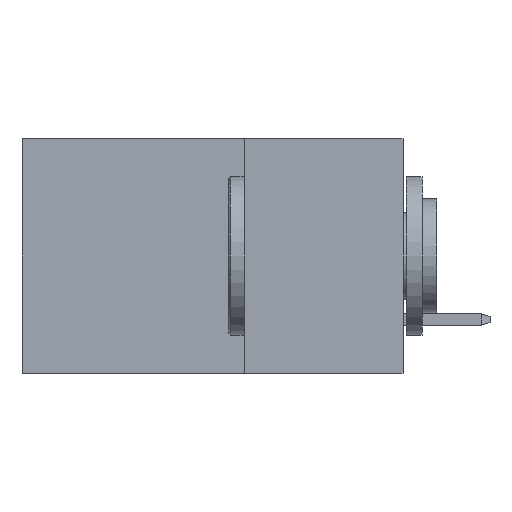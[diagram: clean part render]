
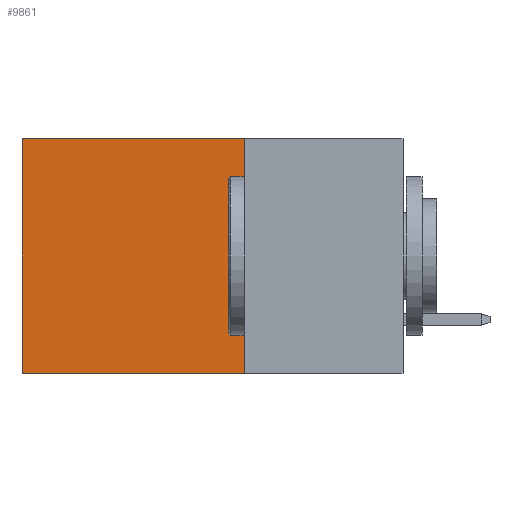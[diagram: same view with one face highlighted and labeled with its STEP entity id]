
A CAD part, left-side view. The second image highlights one B-rep face of the part: STEP entity #9861.
In plain terms, the highlighted planar face has unit normal (-1, 0, 0).
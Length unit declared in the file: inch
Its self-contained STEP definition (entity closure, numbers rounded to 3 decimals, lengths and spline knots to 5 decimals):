
#599 = VERTEX_POINT ( 'NONE', #4474 ) ;
#814 = CARTESIAN_POINT ( 'NONE',  ( 0.2875, 0.25, 0. ) ) ;
#1584 = CARTESIAN_POINT ( 'NONE',  ( 0.2875, 0.6, -0.37 ) ) ;
#2163 = DIRECTION ( 'NONE',  ( 0., 0., -1. ) ) ;
#2333 = LINE ( 'NONE', #814, #4187 ) ;
#2511 = DIRECTION ( 'NONE',  ( 0., 0., -1. ) ) ;
#2760 = CARTESIAN_POINT ( 'NONE',  ( 0.2875, 0.25, 0. ) ) ;
#2828 = EDGE_LOOP ( 'NONE', ( #7615, #7182, #3556, #6015 ) ) ;
#2941 = DIRECTION ( 'NONE',  ( 1., 0., 0. ) ) ;
#2967 = DIRECTION ( 'NONE',  ( 0., 1., 0. ) ) ;
#3556 = ORIENTED_EDGE ( 'NONE', *, *, #6096, .F. ) ;
#3710 = AXIS2_PLACEMENT_3D ( 'NONE', #10039, #2941, #2163 ) ;
#4136 = CARTESIAN_POINT ( 'NONE',  ( 0.2875, 0.6, 0. ) ) ;
#4187 = VECTOR ( 'NONE', #6932, 39.37008 ) ;
#4474 = CARTESIAN_POINT ( 'NONE',  ( 0.2875, 0.25, -0.37 ) ) ;
#4625 = VERTEX_POINT ( 'NONE', #6650 ) ;
#5162 = CARTESIAN_POINT ( 'NONE',  ( 0.2875, 0.6, 0. ) ) ;
#5188 = FACE_OUTER_BOUND ( 'NONE', #2828, .T. ) ;
#5555 = VERTEX_POINT ( 'NONE', #5162 ) ;
#5666 = VECTOR ( 'NONE', #9142, 39.37008 ) ;
#5919 = EDGE_CURVE ( 'NONE', #4625, #5555, #8323, .T. ) ;
#6015 = ORIENTED_EDGE ( 'NONE', *, *, #5919, .T. ) ;
#6096 = EDGE_CURVE ( 'NONE', #4625, #599, #2333, .T. ) ;
#6650 = CARTESIAN_POINT ( 'NONE',  ( 0.2875, 0.25, 0. ) ) ;
#6917 = LINE ( 'NONE', #4136, #7643 ) ;
#6932 = DIRECTION ( 'NONE',  ( 0., 0., -1. ) ) ;
#6945 = CARTESIAN_POINT ( 'NONE',  ( 0.2875, 0.25, -0.37 ) ) ;
#7068 = VERTEX_POINT ( 'NONE', #1584 ) ;
#7182 = ORIENTED_EDGE ( 'NONE', *, *, #8668, .F. ) ;
#7501 = PLANE ( 'NONE',  #3710 ) ;
#7615 = ORIENTED_EDGE ( 'NONE', *, *, #7838, .T. ) ;
#7621 = LINE ( 'NONE', #6945, #9600 ) ;
#7643 = VECTOR ( 'NONE', #2511, 39.37008 ) ;
#7838 = EDGE_CURVE ( 'NONE', #5555, #7068, #6917, .T. ) ;
#8323 = LINE ( 'NONE', #2760, #5666 ) ;
#8668 = EDGE_CURVE ( 'NONE', #599, #7068, #7621, .T. ) ;
#9142 = DIRECTION ( 'NONE',  ( 0., 1., 0. ) ) ;
#9600 = VECTOR ( 'NONE', #2967, 39.37008 ) ;
#9861 = ADVANCED_FACE ( 'NONE', ( #5188 ), #7501, .F. ) ;
#10039 = CARTESIAN_POINT ( 'NONE',  ( 0.2875, 0.25, 0. ) ) ;
